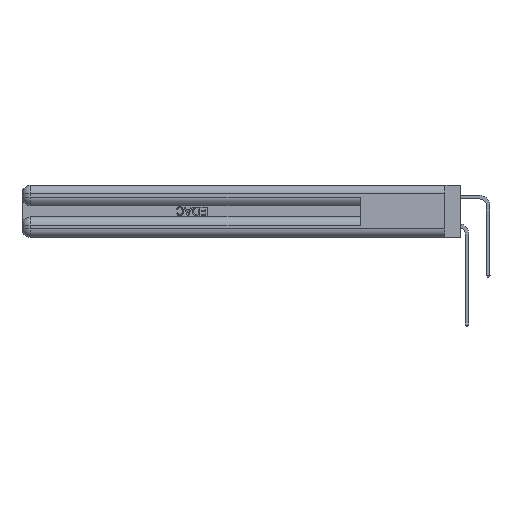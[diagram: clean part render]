
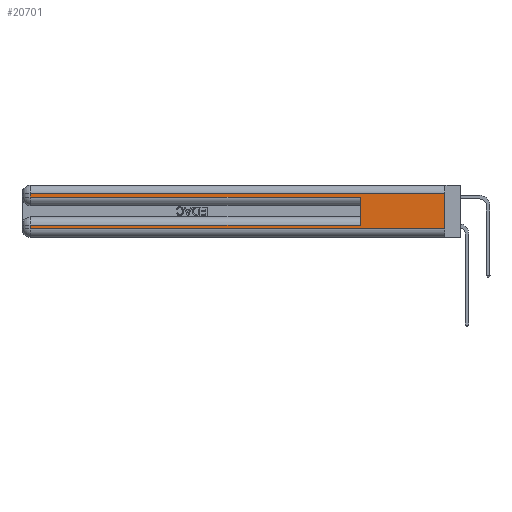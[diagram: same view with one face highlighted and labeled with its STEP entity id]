
A CAD part, left-side view. The second image highlights one B-rep face of the part: STEP entity #20701.
In plain terms, the highlighted planar face has unit normal (-1, 0, 0).
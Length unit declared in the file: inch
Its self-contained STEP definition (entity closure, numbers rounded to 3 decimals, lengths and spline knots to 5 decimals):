
#731 = EDGE_CURVE ( 'NONE', #20438, #3940, #13783, .T. ) ;
#1142 = LINE ( 'NONE', #43201, #40383 ) ;
#2194 = CARTESIAN_POINT ( 'NONE',  ( 0., 0., 0.31 ) ) ;
#2464 = EDGE_CURVE ( 'NONE', #10833, #20438, #8520, .T. ) ;
#2592 = ORIENTED_EDGE ( 'NONE', *, *, #6543, .F. ) ;
#2840 = CARTESIAN_POINT ( 'NONE',  ( 0., 0., 0.37 ) ) ;
#3940 = VERTEX_POINT ( 'NONE', #39563 ) ;
#4196 = VECTOR ( 'NONE', #10520, 39.37008 ) ;
#4457 = CARTESIAN_POINT ( 'NONE',  ( 0., 2.94, 0.285 ) ) ;
#4717 = VERTEX_POINT ( 'NONE', #4866 ) ;
#4740 = LINE ( 'NONE', #2194, #23826 ) ;
#4866 = CARTESIAN_POINT ( 'NONE',  ( 0., 0., 0.06 ) ) ;
#5045 = EDGE_LOOP ( 'NONE', ( #16254, #29389, #30618, #19029, #2592, #36758, #8712, #28370 ) ) ;
#5298 = CARTESIAN_POINT ( 'NONE',  ( 0., 0., 0.37 ) ) ;
#6421 = PLANE ( 'NONE',  #43156 ) ;
#6543 = EDGE_CURVE ( 'NONE', #10833, #36162, #1142, .T. ) ;
#8520 = LINE ( 'NONE', #45850, #45556 ) ;
#8712 = ORIENTED_EDGE ( 'NONE', *, *, #731, .T. ) ;
#10042 = DIRECTION ( 'NONE',  ( 1., 0., 0. ) ) ;
#10091 = DIRECTION ( 'NONE',  ( 0., 1., 0. ) ) ;
#10520 = DIRECTION ( 'NONE',  ( 0., 0., -1. ) ) ;
#10833 = VERTEX_POINT ( 'NONE', #29615 ) ;
#11968 = EDGE_CURVE ( 'NONE', #14851, #30886, #45081, .T. ) ;
#12673 = CARTESIAN_POINT ( 'NONE',  ( 0., 2.94, 0.31 ) ) ;
#13783 = LINE ( 'NONE', #14152, #4196 ) ;
#14048 = VECTOR ( 'NONE', #38485, 39.37008 ) ;
#14152 = CARTESIAN_POINT ( 'NONE',  ( 0., 2.94, 0.37 ) ) ;
#14707 = DIRECTION ( 'NONE',  ( 0., 0., 1. ) ) ;
#14851 = VERTEX_POINT ( 'NONE', #12673 ) ;
#15038 = EDGE_CURVE ( 'NONE', #30886, #36162, #42606, .T. ) ;
#15720 = CARTESIAN_POINT ( 'NONE',  ( 0., 2.94, 0.085 ) ) ;
#15890 = VECTOR ( 'NONE', #25881, 39.37008 ) ;
#16254 = ORIENTED_EDGE ( 'NONE', *, *, #42694, .F. ) ;
#17613 = VECTOR ( 'NONE', #39198, 39.37008 ) ;
#19029 = ORIENTED_EDGE ( 'NONE', *, *, #15038, .T. ) ;
#19354 = CARTESIAN_POINT ( 'NONE',  ( 0., 0., 0.31 ) ) ;
#20438 = VERTEX_POINT ( 'NONE', #15720 ) ;
#20701 = ADVANCED_FACE ( 'NONE', ( #33694 ), #6421, .F. ) ;
#23826 = VECTOR ( 'NONE', #34304, 39.37008 ) ;
#25881 = DIRECTION ( 'NONE',  ( 0., -1., 0. ) ) ;
#27108 = CARTESIAN_POINT ( 'NONE',  ( 0., 0.6, 0.285 ) ) ;
#28370 = ORIENTED_EDGE ( 'NONE', *, *, #46199, .T. ) ;
#29389 = ORIENTED_EDGE ( 'NONE', *, *, #40967, .T. ) ;
#29615 = CARTESIAN_POINT ( 'NONE',  ( 0., 0.6, 0.085 ) ) ;
#30618 = ORIENTED_EDGE ( 'NONE', *, *, #11968, .T. ) ;
#30721 = VECTOR ( 'NONE', #33969, 39.37008 ) ;
#30886 = VERTEX_POINT ( 'NONE', #4457 ) ;
#31835 = LINE ( 'NONE', #5298, #30721 ) ;
#32709 = LINE ( 'NONE', #43897, #15890 ) ;
#33694 = FACE_OUTER_BOUND ( 'NONE', #5045, .T. ) ;
#33969 = DIRECTION ( 'NONE',  ( 0., 0., -1. ) ) ;
#34304 = DIRECTION ( 'NONE',  ( 0., 1., 0. ) ) ;
#34868 = CARTESIAN_POINT ( 'NONE',  ( 0., 0., 0.285 ) ) ;
#35079 = DIRECTION ( 'NONE',  ( 0., 0., -1. ) ) ;
#36162 = VERTEX_POINT ( 'NONE', #27108 ) ;
#36758 = ORIENTED_EDGE ( 'NONE', *, *, #2464, .T. ) ;
#38485 = DIRECTION ( 'NONE',  ( 0., -1., 0. ) ) ;
#39198 = DIRECTION ( 'NONE',  ( 0., 0., -1. ) ) ;
#39563 = CARTESIAN_POINT ( 'NONE',  ( 0., 2.94, 0.06 ) ) ;
#40138 = VERTEX_POINT ( 'NONE', #19354 ) ;
#40383 = VECTOR ( 'NONE', #14707, 39.37008 ) ;
#40967 = EDGE_CURVE ( 'NONE', #40138, #14851, #4740, .T. ) ;
#42502 = CARTESIAN_POINT ( 'NONE',  ( 0., 2.94, 0.37 ) ) ;
#42606 = LINE ( 'NONE', #34868, #14048 ) ;
#42694 = EDGE_CURVE ( 'NONE', #40138, #4717, #31835, .T. ) ;
#43156 = AXIS2_PLACEMENT_3D ( 'NONE', #2840, #10042, #35079 ) ;
#43201 = CARTESIAN_POINT ( 'NONE',  ( 0., 0.6, 0.145 ) ) ;
#43897 = CARTESIAN_POINT ( 'NONE',  ( 0., 0., 0.06 ) ) ;
#45081 = LINE ( 'NONE', #42502, #17613 ) ;
#45556 = VECTOR ( 'NONE', #10091, 39.37008 ) ;
#45850 = CARTESIAN_POINT ( 'NONE',  ( 0., 0., 0.085 ) ) ;
#46199 = EDGE_CURVE ( 'NONE', #3940, #4717, #32709, .T. ) ;
